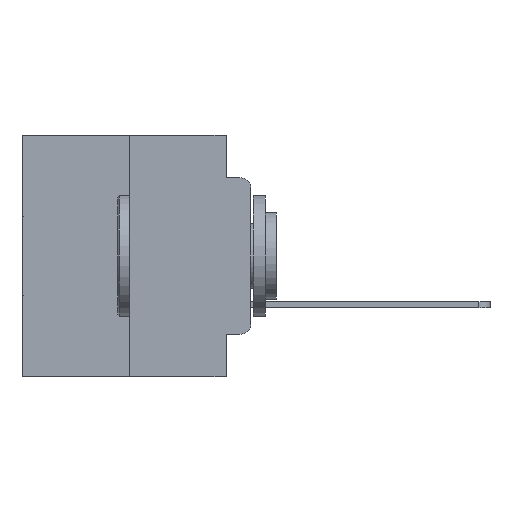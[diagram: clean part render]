
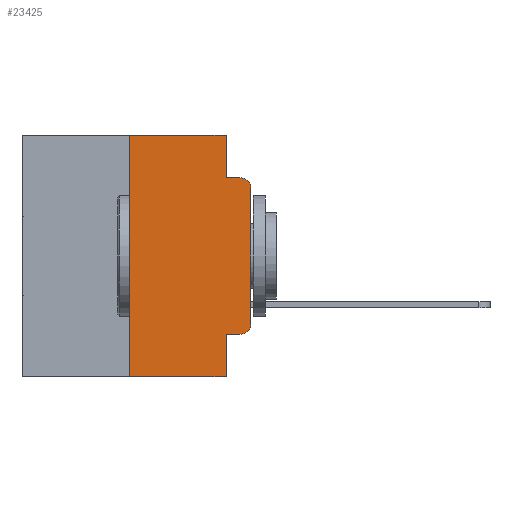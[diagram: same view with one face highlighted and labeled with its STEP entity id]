
A CAD part, left-side view. The second image highlights one B-rep face of the part: STEP entity #23425.
In plain terms, the highlighted planar face has unit normal (-1, 0, 0).
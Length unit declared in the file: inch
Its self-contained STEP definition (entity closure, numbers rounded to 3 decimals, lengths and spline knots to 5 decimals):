
#8 = VERTEX_POINT ( 'NONE', #14423 ) ;
#446 = DIRECTION ( 'NONE',  ( 0., -1., 0. ) ) ;
#837 = ORIENTED_EDGE ( 'NONE', *, *, #10380, .F. ) ;
#1003 = DIRECTION ( 'NONE',  ( 1., 0., 0. ) ) ;
#1233 = VECTOR ( 'NONE', #23118, 39.37008 ) ;
#1307 = EDGE_CURVE ( 'NONE', #8, #27040, #10855, .T. ) ;
#1691 = VERTEX_POINT ( 'NONE', #2851 ) ;
#2074 = CARTESIAN_POINT ( 'NONE',  ( 0., 0.051, 0. ) ) ;
#2149 = LINE ( 'NONE', #21146, #10776 ) ;
#2462 = CARTESIAN_POINT ( 'NONE',  ( 0., 0.473, -0.5 ) ) ;
#2474 = LINE ( 'NONE', #13346, #8144 ) ;
#2809 = VECTOR ( 'NONE', #12196, 39.37008 ) ;
#2851 = CARTESIAN_POINT ( 'NONE',  ( 0., 0.25, -0.5 ) ) ;
#3532 = LINE ( 'NONE', #2462, #4319 ) ;
#3751 = ORIENTED_EDGE ( 'NONE', *, *, #8204, .F. ) ;
#3759 = VERTEX_POINT ( 'NONE', #4764 ) ;
#4255 = ORIENTED_EDGE ( 'NONE', *, *, #12524, .T. ) ;
#4319 = VECTOR ( 'NONE', #18688, 39.37008 ) ;
#4764 = CARTESIAN_POINT ( 'NONE',  ( 0., 0.02, -0.0885 ) ) ;
#5195 = CARTESIAN_POINT ( 'NONE',  ( 0., 0.051, 0. ) ) ;
#5629 = EDGE_CURVE ( 'NONE', #19069, #14261, #20575, .T. ) ;
#5978 = CARTESIAN_POINT ( 'NONE',  ( 0., 0.051, -0.0885 ) ) ;
#6034 = CARTESIAN_POINT ( 'NONE',  ( 0., 0., -0.1085 ) ) ;
#6065 = CARTESIAN_POINT ( 'NONE',  ( 0., 0.25, 0. ) ) ;
#6195 = DIRECTION ( 'NONE',  ( -1., 0., 0. ) ) ;
#6414 = DIRECTION ( 'NONE',  ( 0., -1., 0. ) ) ;
#6475 = LINE ( 'NONE', #19039, #23160 ) ;
#7274 = CARTESIAN_POINT ( 'NONE',  ( 0., 0.051, -0.0885 ) ) ;
#7611 = DIRECTION ( 'NONE',  ( 0., 0., 1. ) ) ;
#7894 = VERTEX_POINT ( 'NONE', #6065 ) ;
#8144 = VECTOR ( 'NONE', #20018, 39.37008 ) ;
#8169 = LINE ( 'NONE', #17798, #19493 ) ;
#8204 = EDGE_CURVE ( 'NONE', #27448, #3759, #25017, .T. ) ;
#8775 = ORIENTED_EDGE ( 'NONE', *, *, #5629, .F. ) ;
#10380 = EDGE_CURVE ( 'NONE', #1691, #7894, #2149, .T. ) ;
#10633 = ORIENTED_EDGE ( 'NONE', *, *, #19930, .T. ) ;
#10776 = VECTOR ( 'NONE', #7611, 39.37008 ) ;
#10836 = CARTESIAN_POINT ( 'NONE',  ( 0., 0., -0.3915 ) ) ;
#10855 = CIRCLE ( 'NONE', #13502, 0.02 ) ;
#11761 = CARTESIAN_POINT ( 'NONE',  ( 0., 0.051, 0. ) ) ;
#12196 = DIRECTION ( 'NONE',  ( 0., 0., -1. ) ) ;
#12258 = VERTEX_POINT ( 'NONE', #6034 ) ;
#12502 = DIRECTION ( 'NONE',  ( 0., 0., -1. ) ) ;
#12524 = EDGE_CURVE ( 'NONE', #1691, #14261, #3532, .T. ) ;
#12769 = CIRCLE ( 'NONE', #29160, 0.02 ) ;
#12888 = EDGE_CURVE ( 'NONE', #12258, #3759, #12769, .T. ) ;
#13346 = CARTESIAN_POINT ( 'NONE',  ( 0., 0., 0. ) ) ;
#13502 = AXIS2_PLACEMENT_3D ( 'NONE', #21513, #17673, #12502 ) ;
#13985 = DIRECTION ( 'NONE',  ( 0., 0., -1. ) ) ;
#14261 = VERTEX_POINT ( 'NONE', #20513 ) ;
#14423 = CARTESIAN_POINT ( 'NONE',  ( 0., 0.02, -0.4115 ) ) ;
#14688 = VECTOR ( 'NONE', #13985, 39.37008 ) ;
#14788 = FACE_OUTER_BOUND ( 'NONE', #26979, .T. ) ;
#15157 = PLANE ( 'NONE',  #18498 ) ;
#16369 = EDGE_CURVE ( 'NONE', #7894, #20115, #6475, .T. ) ;
#17364 = DIRECTION ( 'NONE',  ( 0., 0., -1. ) ) ;
#17631 = ORIENTED_EDGE ( 'NONE', *, *, #1307, .T. ) ;
#17673 = DIRECTION ( 'NONE',  ( -1., 0., 0. ) ) ;
#17798 = CARTESIAN_POINT ( 'NONE',  ( 0., 0.051, -0.4115 ) ) ;
#18498 = AXIS2_PLACEMENT_3D ( 'NONE', #28278, #1003, #17364 ) ;
#18688 = DIRECTION ( 'NONE',  ( 0., -1., 0. ) ) ;
#19039 = CARTESIAN_POINT ( 'NONE',  ( 0., 0.473, 0. ) ) ;
#19069 = VERTEX_POINT ( 'NONE', #19983 ) ;
#19493 = VECTOR ( 'NONE', #6414, 39.37008 ) ;
#19800 = CARTESIAN_POINT ( 'NONE',  ( 0., 0.02, -0.1085 ) ) ;
#19930 = EDGE_CURVE ( 'NONE', #19069, #8, #8169, .T. ) ;
#19983 = CARTESIAN_POINT ( 'NONE',  ( 0., 0.051, -0.4115 ) ) ;
#20018 = DIRECTION ( 'NONE',  ( 0., 0., 1. ) ) ;
#20115 = VERTEX_POINT ( 'NONE', #11761 ) ;
#20513 = CARTESIAN_POINT ( 'NONE',  ( 0., 0.051, -0.5 ) ) ;
#20575 = LINE ( 'NONE', #2074, #14688 ) ;
#20882 = EDGE_CURVE ( 'NONE', #20115, #27448, #27104, .T. ) ;
#21146 = CARTESIAN_POINT ( 'NONE',  ( 0., 0.25, 0. ) ) ;
#21513 = CARTESIAN_POINT ( 'NONE',  ( 0., 0.02, -0.3915 ) ) ;
#22057 = DIRECTION ( 'NONE',  ( 0., 0., -1. ) ) ;
#23097 = ORIENTED_EDGE ( 'NONE', *, *, #20882, .F. ) ;
#23118 = DIRECTION ( 'NONE',  ( 0., -1., 0. ) ) ;
#23160 = VECTOR ( 'NONE', #446, 39.37008 ) ;
#23425 = ADVANCED_FACE ( 'NONE', ( #14788 ), #15157, .F. ) ;
#24050 = ORIENTED_EDGE ( 'NONE', *, *, #26302, .T. ) ;
#25017 = LINE ( 'NONE', #7274, #1233 ) ;
#26302 = EDGE_CURVE ( 'NONE', #27040, #12258, #2474, .T. ) ;
#26504 = ORIENTED_EDGE ( 'NONE', *, *, #12888, .T. ) ;
#26926 = ORIENTED_EDGE ( 'NONE', *, *, #16369, .F. ) ;
#26979 = EDGE_LOOP ( 'NONE', ( #24050, #26504, #3751, #23097, #26926, #837, #4255, #8775, #10633, #17631 ) ) ;
#27040 = VERTEX_POINT ( 'NONE', #10836 ) ;
#27104 = LINE ( 'NONE', #5195, #2809 ) ;
#27448 = VERTEX_POINT ( 'NONE', #5978 ) ;
#28278 = CARTESIAN_POINT ( 'NONE',  ( 0., 0.473, 0. ) ) ;
#29160 = AXIS2_PLACEMENT_3D ( 'NONE', #19800, #6195, #22057 ) ;
